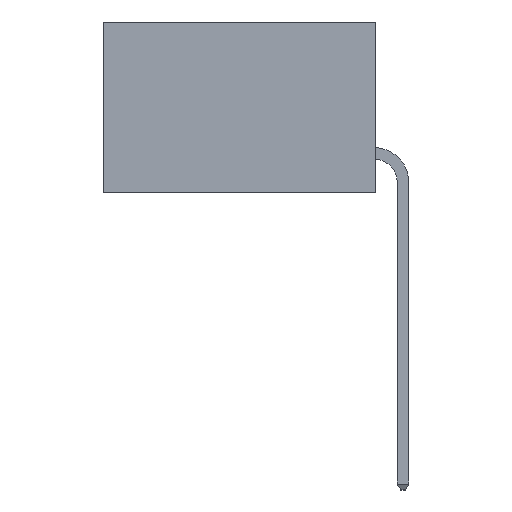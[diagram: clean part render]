
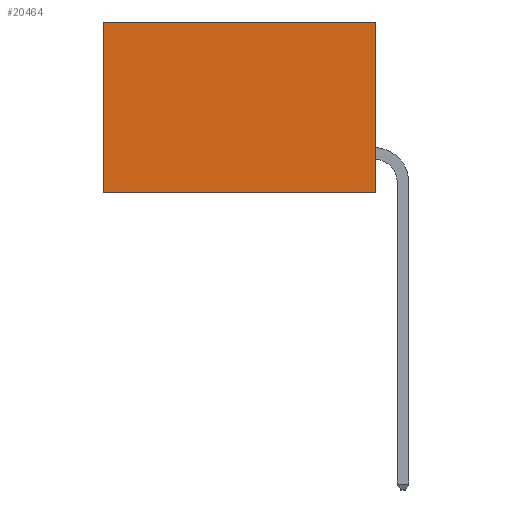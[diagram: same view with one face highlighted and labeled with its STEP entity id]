
A CAD part, left-side view. The second image highlights one B-rep face of the part: STEP entity #20464.
In plain terms, the highlighted planar face has unit normal (-1, 0, 0).
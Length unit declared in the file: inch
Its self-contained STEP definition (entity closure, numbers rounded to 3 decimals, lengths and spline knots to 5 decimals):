
#618 = VERTEX_POINT ( 'NONE', #20687 ) ;
#907 = ORIENTED_EDGE ( 'NONE', *, *, #17347, .F. ) ;
#1299 = EDGE_CURVE ( 'NONE', #8467, #21564, #11694, .T. ) ;
#1655 = DIRECTION ( 'NONE',  ( 0., 1., 0. ) ) ;
#1906 = DIRECTION ( 'NONE',  ( 0., 1., 0. ) ) ;
#2985 = VECTOR ( 'NONE', #1655, 39.37008 ) ;
#3756 = CARTESIAN_POINT ( 'NONE',  ( 0.277, 0., 0. ) ) ;
#5427 = VECTOR ( 'NONE', #7152, 39.37008 ) ;
#5544 = CARTESIAN_POINT ( 'NONE',  ( 0.277, 0.59, -0.37 ) ) ;
#5557 = ORIENTED_EDGE ( 'NONE', *, *, #1299, .T. ) ;
#6854 = ORIENTED_EDGE ( 'NONE', *, *, #21254, .T. ) ;
#7152 = DIRECTION ( 'NONE',  ( 0., 0., -1. ) ) ;
#8467 = VERTEX_POINT ( 'NONE', #15861 ) ;
#8607 = CARTESIAN_POINT ( 'NONE',  ( 0.277, 0., -0.37 ) ) ;
#9142 = LINE ( 'NONE', #13975, #17610 ) ;
#9596 = CARTESIAN_POINT ( 'NONE',  ( 0.277, 0., -0.37 ) ) ;
#10359 = DIRECTION ( 'NONE',  ( 0., 0., -1. ) ) ;
#11694 = LINE ( 'NONE', #3756, #2985 ) ;
#11959 = VECTOR ( 'NONE', #21408, 39.37008 ) ;
#12830 = ORIENTED_EDGE ( 'NONE', *, *, #16390, .F. ) ;
#13975 = CARTESIAN_POINT ( 'NONE',  ( 0.277, 0., -0.37 ) ) ;
#14113 = EDGE_LOOP ( 'NONE', ( #6854, #907, #12830, #5557 ) ) ;
#14136 = FACE_OUTER_BOUND ( 'NONE', #14113, .T. ) ;
#15095 = LINE ( 'NONE', #20717, #5427 ) ;
#15861 = CARTESIAN_POINT ( 'NONE',  ( 0.277, 0., 0. ) ) ;
#16390 = EDGE_CURVE ( 'NONE', #8467, #618, #20774, .T. ) ;
#17347 = EDGE_CURVE ( 'NONE', #618, #18739, #9142, .T. ) ;
#17610 = VECTOR ( 'NONE', #1906, 39.37008 ) ;
#18715 = PLANE ( 'NONE',  #20702 ) ;
#18739 = VERTEX_POINT ( 'NONE', #5544 ) ;
#20390 = DIRECTION ( 'NONE',  ( 1., 0., 0. ) ) ;
#20464 = ADVANCED_FACE ( 'NONE', ( #14136 ), #18715, .F. ) ;
#20687 = CARTESIAN_POINT ( 'NONE',  ( 0.277, 0., -0.37 ) ) ;
#20702 = AXIS2_PLACEMENT_3D ( 'NONE', #8607, #20390, #10359 ) ;
#20717 = CARTESIAN_POINT ( 'NONE',  ( 0.277, 0.59, -0.37 ) ) ;
#20774 = LINE ( 'NONE', #9596, #11959 ) ;
#21254 = EDGE_CURVE ( 'NONE', #21564, #18739, #15095, .T. ) ;
#21408 = DIRECTION ( 'NONE',  ( 0., 0., -1. ) ) ;
#21420 = CARTESIAN_POINT ( 'NONE',  ( 0.277, 0.59, 0. ) ) ;
#21564 = VERTEX_POINT ( 'NONE', #21420 ) ;
